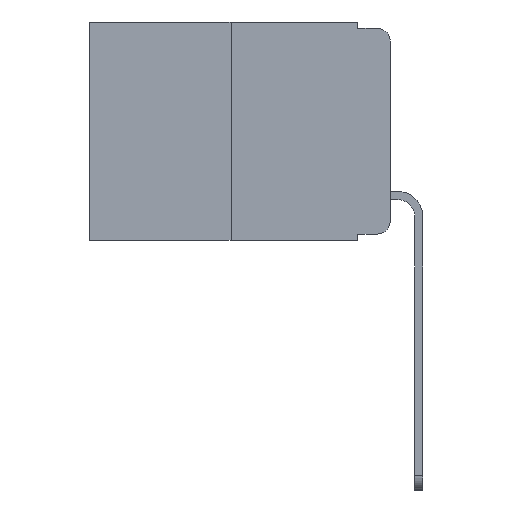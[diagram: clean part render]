
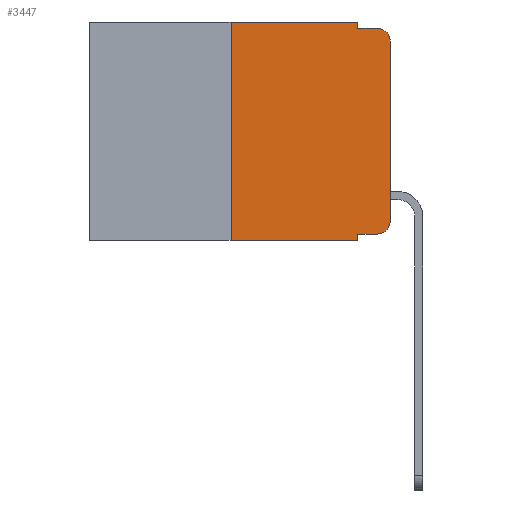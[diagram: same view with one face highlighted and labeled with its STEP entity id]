
A CAD part, left-side view. The second image highlights one B-rep face of the part: STEP entity #3447.
In plain terms, the highlighted planar face has unit normal (-1, 0, 0).
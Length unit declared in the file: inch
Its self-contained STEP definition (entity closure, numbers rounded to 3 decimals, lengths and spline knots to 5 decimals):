
#135 = VECTOR ( 'NONE', #7009, 39.37008 ) ;
#493 = VERTEX_POINT ( 'NONE', #11196 ) ;
#499 = DIRECTION ( 'NONE',  ( 0., 0., -1. ) ) ;
#746 = VECTOR ( 'NONE', #2124, 39.37008 ) ;
#783 = ORIENTED_EDGE ( 'NONE', *, *, #9330, .T. ) ;
#1018 = ORIENTED_EDGE ( 'NONE', *, *, #13521, .F. ) ;
#1313 = ORIENTED_EDGE ( 'NONE', *, *, #7120, .F. ) ;
#1456 = CARTESIAN_POINT ( 'NONE',  ( 0., 0.473, 0. ) ) ;
#1508 = ORIENTED_EDGE ( 'NONE', *, *, #5771, .T. ) ;
#2087 = VECTOR ( 'NONE', #4697, 39.37008 ) ;
#2124 = DIRECTION ( 'NONE',  ( 0., 0., -1. ) ) ;
#2237 = ORIENTED_EDGE ( 'NONE', *, *, #12211, .F. ) ;
#2390 = CARTESIAN_POINT ( 'NONE',  ( 0., 0.25, -0.343 ) ) ;
#2482 = ORIENTED_EDGE ( 'NONE', *, *, #7935, .T. ) ;
#2508 = CARTESIAN_POINT ( 'NONE',  ( 0., 0.051, 0. ) ) ;
#2666 = VERTEX_POINT ( 'NONE', #2508 ) ;
#2905 = VECTOR ( 'NONE', #10070, 39.37008 ) ;
#2927 = EDGE_CURVE ( 'NONE', #11410, #493, #11226, .T. ) ;
#2966 = ORIENTED_EDGE ( 'NONE', *, *, #2927, .F. ) ;
#3126 = CARTESIAN_POINT ( 'NONE',  ( 0., 0.051, -0.333 ) ) ;
#3136 = AXIS2_PLACEMENT_3D ( 'NONE', #13064, #7037, #499 ) ;
#3237 = VERTEX_POINT ( 'NONE', #7933 ) ;
#3265 = EDGE_LOOP ( 'NONE', ( #783, #2482, #2966, #1018, #1313, #2237, #1508, #12048, #8895, #12986 ) ) ;
#3447 = ADVANCED_FACE ( 'NONE', ( #4731 ), #10316, .F. ) ;
#4649 = CARTESIAN_POINT ( 'NONE',  ( 0., 0.473, -0.343 ) ) ;
#4697 = DIRECTION ( 'NONE',  ( 0., -1., 0. ) ) ;
#4731 = FACE_OUTER_BOUND ( 'NONE', #3265, .T. ) ;
#4866 = CARTESIAN_POINT ( 'NONE',  ( 0., 0., 0. ) ) ;
#5011 = VECTOR ( 'NONE', #6377, 39.37008 ) ;
#5098 = DIRECTION ( 'NONE',  ( 1., 0., 0. ) ) ;
#5106 = VERTEX_POINT ( 'NONE', #7831 ) ;
#5160 = VECTOR ( 'NONE', #12515, 39.37008 ) ;
#5252 = DIRECTION ( 'NONE',  ( 0., -1., 0. ) ) ;
#5503 = LINE ( 'NONE', #10563, #5160 ) ;
#5660 = VERTEX_POINT ( 'NONE', #9774 ) ;
#5771 = EDGE_CURVE ( 'NONE', #6330, #5106, #13130, .T. ) ;
#5974 = CARTESIAN_POINT ( 'NONE',  ( 0., 0.02, -0.03 ) ) ;
#6215 = CARTESIAN_POINT ( 'NONE',  ( 0., 0.02, -0.333 ) ) ;
#6266 = VERTEX_POINT ( 'NONE', #12707 ) ;
#6330 = VERTEX_POINT ( 'NONE', #2390 ) ;
#6377 = DIRECTION ( 'NONE',  ( 0., -1., 0. ) ) ;
#7009 = DIRECTION ( 'NONE',  ( 0., 0., 1. ) ) ;
#7030 = DIRECTION ( 'NONE',  ( 0., 0., -1. ) ) ;
#7037 = DIRECTION ( 'NONE',  ( -1., 0., 0. ) ) ;
#7120 = EDGE_CURVE ( 'NONE', #7424, #2666, #12320, .T. ) ;
#7424 = VERTEX_POINT ( 'NONE', #10353 ) ;
#7831 = CARTESIAN_POINT ( 'NONE',  ( 0., 0.051, -0.343 ) ) ;
#7933 = CARTESIAN_POINT ( 'NONE',  ( 0., 0., -0.03 ) ) ;
#7935 = EDGE_CURVE ( 'NONE', #3237, #493, #13392, .T. ) ;
#7986 = CARTESIAN_POINT ( 'NONE',  ( 0., 0.25, 0. ) ) ;
#8191 = EDGE_CURVE ( 'NONE', #13396, #5660, #11256, .T. ) ;
#8895 = ORIENTED_EDGE ( 'NONE', *, *, #8901, .T. ) ;
#8901 = EDGE_CURVE ( 'NONE', #6266, #13396, #13149, .T. ) ;
#8982 = DIRECTION ( 'NONE',  ( 0., -1., 0. ) ) ;
#9112 = AXIS2_PLACEMENT_3D ( 'NONE', #5974, #13057, #7030 ) ;
#9294 = CARTESIAN_POINT ( 'NONE',  ( 0., 0.473, 0. ) ) ;
#9330 = EDGE_CURVE ( 'NONE', #5660, #3237, #11462, .T. ) ;
#9591 = EDGE_CURVE ( 'NONE', #6266, #5106, #5503, .T. ) ;
#9774 = CARTESIAN_POINT ( 'NONE',  ( 0., 0., -0.313 ) ) ;
#10070 = DIRECTION ( 'NONE',  ( 0., 0., 1. ) ) ;
#10316 = PLANE ( 'NONE',  #10890 ) ;
#10353 = CARTESIAN_POINT ( 'NONE',  ( 0., 0.25, 0. ) ) ;
#10457 = CARTESIAN_POINT ( 'NONE',  ( 0., 0.051, -0.01 ) ) ;
#10563 = CARTESIAN_POINT ( 'NONE',  ( 0., 0.051, 0. ) ) ;
#10590 = CARTESIAN_POINT ( 'NONE',  ( 0., 0.051, 0. ) ) ;
#10890 = AXIS2_PLACEMENT_3D ( 'NONE', #9294, #5098, #12256 ) ;
#10918 = VECTOR ( 'NONE', #5252, 39.37008 ) ;
#11095 = CARTESIAN_POINT ( 'NONE',  ( 0., 0.051, -0.01 ) ) ;
#11196 = CARTESIAN_POINT ( 'NONE',  ( 0., 0.02, -0.01 ) ) ;
#11226 = LINE ( 'NONE', #10457, #10918 ) ;
#11256 = CIRCLE ( 'NONE', #3136, 0.02 ) ;
#11410 = VERTEX_POINT ( 'NONE', #11095 ) ;
#11462 = LINE ( 'NONE', #4866, #135 ) ;
#11665 = LINE ( 'NONE', #10590, #746 ) ;
#11711 = VECTOR ( 'NONE', #8982, 39.37008 ) ;
#12048 = ORIENTED_EDGE ( 'NONE', *, *, #9591, .F. ) ;
#12211 = EDGE_CURVE ( 'NONE', #6330, #7424, #13524, .T. ) ;
#12256 = DIRECTION ( 'NONE',  ( 0., 0., -1. ) ) ;
#12320 = LINE ( 'NONE', #1456, #11711 ) ;
#12515 = DIRECTION ( 'NONE',  ( 0., 0., -1. ) ) ;
#12707 = CARTESIAN_POINT ( 'NONE',  ( 0., 0.051, -0.333 ) ) ;
#12986 = ORIENTED_EDGE ( 'NONE', *, *, #8191, .T. ) ;
#13057 = DIRECTION ( 'NONE',  ( -1., 0., 0. ) ) ;
#13064 = CARTESIAN_POINT ( 'NONE',  ( 0., 0.02, -0.313 ) ) ;
#13130 = LINE ( 'NONE', #4649, #2087 ) ;
#13149 = LINE ( 'NONE', #3126, #5011 ) ;
#13392 = CIRCLE ( 'NONE', #9112, 0.02 ) ;
#13396 = VERTEX_POINT ( 'NONE', #6215 ) ;
#13521 = EDGE_CURVE ( 'NONE', #2666, #11410, #11665, .T. ) ;
#13524 = LINE ( 'NONE', #7986, #2905 ) ;
